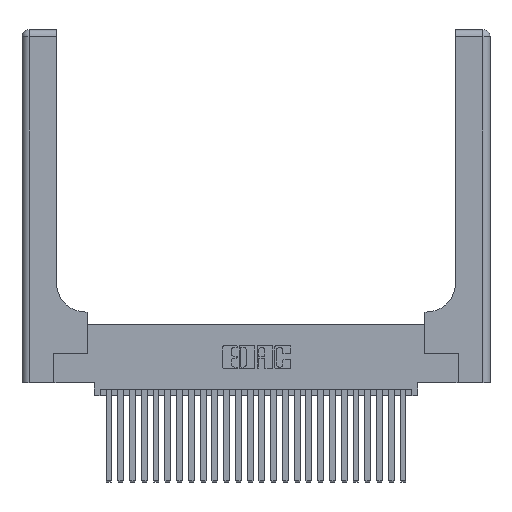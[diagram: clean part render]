
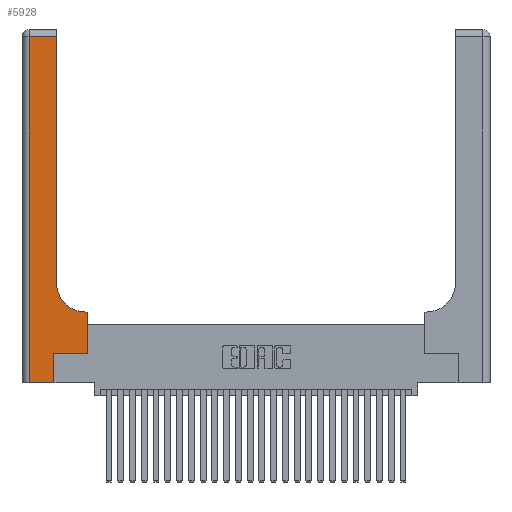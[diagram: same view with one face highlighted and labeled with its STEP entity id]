
A CAD part, top view. The second image highlights one B-rep face of the part: STEP entity #5928.
In plain terms, the highlighted planar face has unit normal (0, 0, 1).
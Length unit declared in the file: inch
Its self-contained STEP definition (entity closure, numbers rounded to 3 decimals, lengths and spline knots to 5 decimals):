
#330 = CARTESIAN_POINT ( 'NONE',  ( 0.5585, 0.25, 0.37 ) ) ;
#669 = ORIENTED_EDGE ( 'NONE', *, *, #21359, .T. ) ;
#1572 = EDGE_LOOP ( 'NONE', ( #6106, #669, #7043, #8587, #22958, #9842, #17952, #11153, #10437 ) ) ;
#2055 = EDGE_CURVE ( 'NONE', #10759, #17622, #25330, .T. ) ;
#2124 = CARTESIAN_POINT ( 'NONE',  ( 0.06, 2.94, 0.37 ) ) ;
#2325 = VECTOR ( 'NONE', #12660, 39.37008 ) ;
#3006 = VECTOR ( 'NONE', #7660, 39.37008 ) ;
#3129 = CARTESIAN_POINT ( 'NONE',  ( 0.269, 0.25, 0.37 ) ) ;
#3184 = VERTEX_POINT ( 'NONE', #11165 ) ;
#3340 = CARTESIAN_POINT ( 'NONE',  ( 0.269, 0.25, 0.37 ) ) ;
#3458 = LINE ( 'NONE', #15854, #4785 ) ;
#3477 = EDGE_CURVE ( 'NONE', #18405, #3184, #9840, .T. ) ;
#3935 = VECTOR ( 'NONE', #18807, 39.37008 ) ;
#4496 = LINE ( 'NONE', #26702, #14496 ) ;
#4785 = VECTOR ( 'NONE', #20051, 39.37008 ) ;
#4949 = CARTESIAN_POINT ( 'NONE',  ( 0.5585, 0.25, 0.37 ) ) ;
#5928 = ADVANCED_FACE ( 'NONE', ( #14026 ), #7289, .F. ) ;
#5934 = CARTESIAN_POINT ( 'NONE',  ( 0.06, 3., 0.37 ) ) ;
#6106 = ORIENTED_EDGE ( 'NONE', *, *, #25199, .T. ) ;
#6507 = VECTOR ( 'NONE', #14041, 39.37008 ) ;
#7043 = ORIENTED_EDGE ( 'NONE', *, *, #2055, .T. ) ;
#7068 = EDGE_CURVE ( 'NONE', #8686, #9905, #20381, .T. ) ;
#7181 = CARTESIAN_POINT ( 'NONE',  ( 0.2915, 2.94, 0.37 ) ) ;
#7289 = PLANE ( 'NONE',  #7411 ) ;
#7411 = AXIS2_PLACEMENT_3D ( 'NONE', #15661, #27187, #22655 ) ;
#7660 = DIRECTION ( 'NONE',  ( -1., 0., 0. ) ) ;
#7945 = AXIS2_PLACEMENT_3D ( 'NONE', #24610, #11607, #13941 ) ;
#8010 = EDGE_CURVE ( 'NONE', #21911, #25268, #19353, .T. ) ;
#8587 = ORIENTED_EDGE ( 'NONE', *, *, #15906, .T. ) ;
#8686 = VERTEX_POINT ( 'NONE', #9328 ) ;
#9328 = CARTESIAN_POINT ( 'NONE',  ( 0.5415, 0.6, 0.37 ) ) ;
#9840 = LINE ( 'NONE', #4949, #13194 ) ;
#9842 = ORIENTED_EDGE ( 'NONE', *, *, #16456, .T. ) ;
#9905 = VERTEX_POINT ( 'NONE', #27127 ) ;
#10229 = VERTEX_POINT ( 'NONE', #7181 ) ;
#10437 = ORIENTED_EDGE ( 'NONE', *, *, #7068, .T. ) ;
#10759 = VERTEX_POINT ( 'NONE', #2124 ) ;
#11153 = ORIENTED_EDGE ( 'NONE', *, *, #25876, .T. ) ;
#11165 = CARTESIAN_POINT ( 'NONE',  ( 0.5585, 0.6, 0.37 ) ) ;
#11607 = DIRECTION ( 'NONE',  ( 0., 0., -1. ) ) ;
#12660 = DIRECTION ( 'NONE',  ( 0., 1., 0. ) ) ;
#13194 = VECTOR ( 'NONE', #22493, 39.37008 ) ;
#13245 = LINE ( 'NONE', #23887, #21578 ) ;
#13941 = DIRECTION ( 'NONE',  ( 1., 0., 0. ) ) ;
#14026 = FACE_OUTER_BOUND ( 'NONE', #1572, .T. ) ;
#14041 = DIRECTION ( 'NONE',  ( 1., 0., 0. ) ) ;
#14496 = VECTOR ( 'NONE', #18239, 39.37008 ) ;
#15480 = CARTESIAN_POINT ( 'NONE',  ( 0.06, 0., 0.37 ) ) ;
#15661 = CARTESIAN_POINT ( 'NONE',  ( 0., 3., 0.37 ) ) ;
#15854 = CARTESIAN_POINT ( 'NONE',  ( 0.2915, 0.6, 0.37 ) ) ;
#15906 = EDGE_CURVE ( 'NONE', #17622, #21911, #13245, .T. ) ;
#16456 = EDGE_CURVE ( 'NONE', #25268, #18405, #16518, .T. ) ;
#16518 = LINE ( 'NONE', #3129, #6507 ) ;
#16831 = CARTESIAN_POINT ( 'NONE',  ( 0.269, 0., 0.37 ) ) ;
#17298 = DIRECTION ( 'NONE',  ( 1., 0., 0. ) ) ;
#17622 = VERTEX_POINT ( 'NONE', #15480 ) ;
#17952 = ORIENTED_EDGE ( 'NONE', *, *, #3477, .T. ) ;
#18239 = DIRECTION ( 'NONE',  ( 0., 1., 0. ) ) ;
#18405 = VERTEX_POINT ( 'NONE', #330 ) ;
#18807 = DIRECTION ( 'NONE',  ( 0., -1., 0. ) ) ;
#19353 = LINE ( 'NONE', #16831, #2325 ) ;
#20012 = LINE ( 'NONE', #24642, #3006 ) ;
#20051 = DIRECTION ( 'NONE',  ( -1., 0., 0. ) ) ;
#20381 = CIRCLE ( 'NONE', #7945, 0.25 ) ;
#21359 = EDGE_CURVE ( 'NONE', #10229, #10759, #20012, .T. ) ;
#21578 = VECTOR ( 'NONE', #17298, 39.37008 ) ;
#21911 = VERTEX_POINT ( 'NONE', #22520 ) ;
#22493 = DIRECTION ( 'NONE',  ( 0., 1., 0. ) ) ;
#22520 = CARTESIAN_POINT ( 'NONE',  ( 0.269, 0., 0.37 ) ) ;
#22655 = DIRECTION ( 'NONE',  ( -1., 0., 0. ) ) ;
#22958 = ORIENTED_EDGE ( 'NONE', *, *, #8010, .T. ) ;
#23887 = CARTESIAN_POINT ( 'NONE',  ( 0., 0., 0.37 ) ) ;
#24610 = CARTESIAN_POINT ( 'NONE',  ( 0.5415, 0.85, 0.37 ) ) ;
#24642 = CARTESIAN_POINT ( 'NONE',  ( 0., 2.94, 0.37 ) ) ;
#25199 = EDGE_CURVE ( 'NONE', #9905, #10229, #4496, .T. ) ;
#25268 = VERTEX_POINT ( 'NONE', #3340 ) ;
#25330 = LINE ( 'NONE', #5934, #3935 ) ;
#25876 = EDGE_CURVE ( 'NONE', #3184, #8686, #3458, .T. ) ;
#26702 = CARTESIAN_POINT ( 'NONE',  ( 0.2915, 3., 0.37 ) ) ;
#27127 = CARTESIAN_POINT ( 'NONE',  ( 0.2915, 0.85, 0.37 ) ) ;
#27187 = DIRECTION ( 'NONE',  ( 0., 0., -1. ) ) ;
